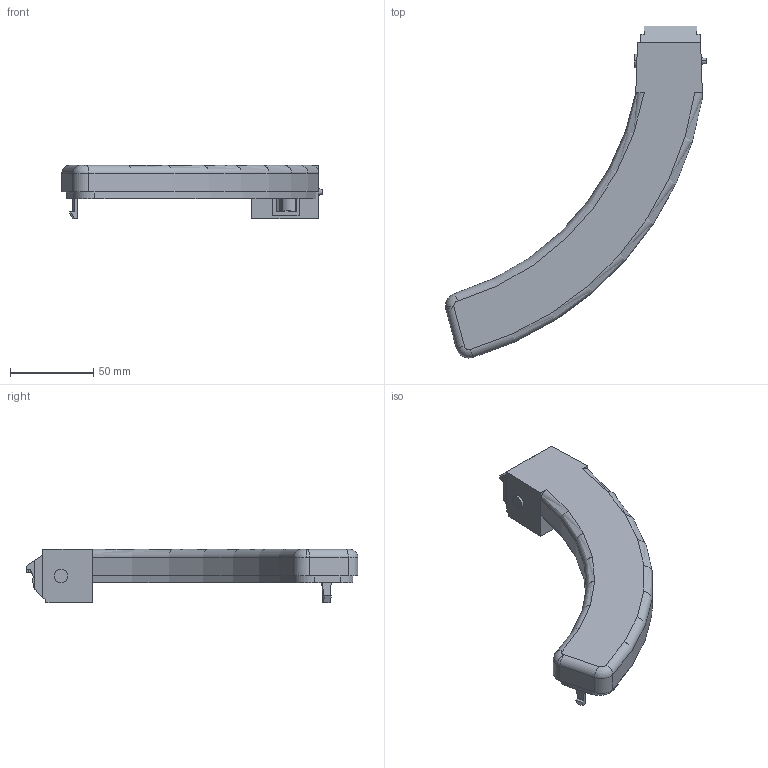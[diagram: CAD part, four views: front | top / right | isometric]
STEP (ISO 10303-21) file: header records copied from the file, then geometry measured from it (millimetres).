
FILE_DESCRIPTION (( 'STEP AP214' ), '1' );
FILE_NAME ('right_large.STEP', '2013-07-01T00:24:44', ( '' ), ( '' ), 'SwSTEP 2.0', 'SolidWorks 2013', '' );
FILE_SCHEMA (( 'AUTOMOTIVE_DESIGN' ));
Length unit declared in the file: millimetre
Products named in the file (1): right_large
Bounding box: 156.86 x 199.55 x 32 mm (x, y, z)
Volume: 100611 mm3; surface area: 53865.8 mm2
Topology: 1 solids, 1 shells, 199 faces, 559 edges, 366 vertices
Faces by surface type: plane 127, cylinder 57, torus 10, bspline 3, cone 2
Entity records: 6617 total; most frequent: CARTESIAN_POINT 1396, ORIENTED_EDGE 1118, DIRECTION 1074, EDGE_CURVE 559, LINE 368, VECTOR 368, VERTEX_POINT 366, AXIS2_PLACEMENT_3D 353
